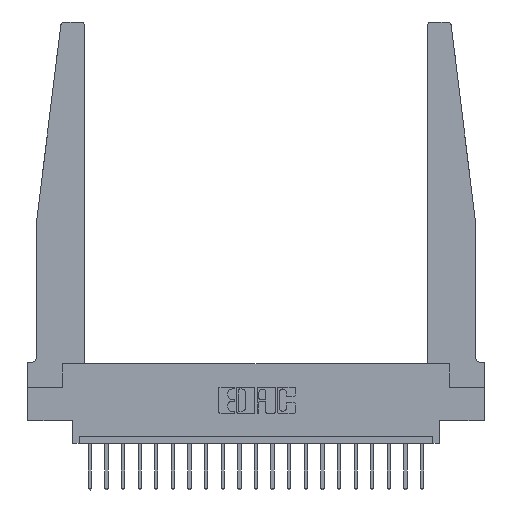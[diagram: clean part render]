
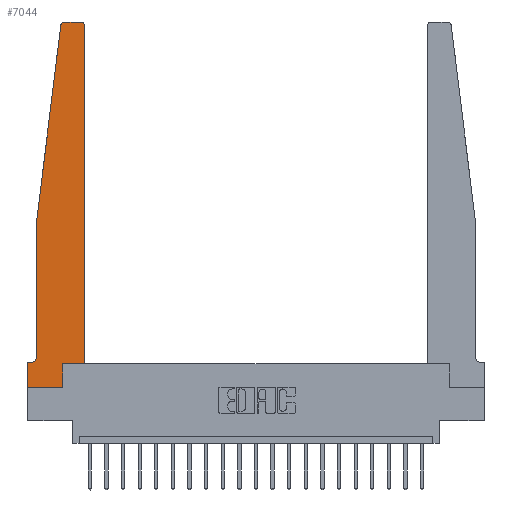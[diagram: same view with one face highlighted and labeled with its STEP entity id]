
A CAD part, top view. The second image highlights one B-rep face of the part: STEP entity #7044.
In plain terms, the highlighted planar face has unit normal (0, 0, 1).
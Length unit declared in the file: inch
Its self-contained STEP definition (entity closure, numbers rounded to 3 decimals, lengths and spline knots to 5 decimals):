
#80 = DIRECTION ( 'NONE',  ( 1., 0., 0. ) ) ;
#174 = VECTOR ( 'NONE', #80, 39.37008 ) ;
#444 = EDGE_CURVE ( 'NONE', #9945, #9003, #4752, .T. ) ;
#501 = CARTESIAN_POINT ( 'NONE',  ( 0.425, 0.18, 0.37 ) ) ;
#555 = EDGE_CURVE ( 'NONE', #20410, #11046, #13767, .T. ) ;
#638 = ORIENTED_EDGE ( 'NONE', *, *, #2911, .T. ) ;
#1196 = DIRECTION ( 'NONE',  ( -1., 0., 0. ) ) ;
#1366 = CIRCLE ( 'NONE', #17607, 0.05 ) ;
#1456 = EDGE_CURVE ( 'NONE', #18994, #9248, #15527, .T. ) ;
#1586 = CARTESIAN_POINT ( 'NONE',  ( 0.015, 0.2375, 0.37 ) ) ;
#1718 = CARTESIAN_POINT ( 'NONE',  ( 0.2605, 0.18, 0.37 ) ) ;
#1990 = DIRECTION ( 'NONE',  ( 0., 0., 1. ) ) ;
#2116 = CARTESIAN_POINT ( 'NONE',  ( 0.065, 1.25, 0.37 ) ) ;
#2393 = LINE ( 'NONE', #12833, #174 ) ;
#2533 = EDGE_CURVE ( 'NONE', #6152, #16121, #2393, .T. ) ;
#2654 = CARTESIAN_POINT ( 'NONE',  ( 0.065, 0.2375, 0.37 ) ) ;
#2911 = EDGE_CURVE ( 'NONE', #16121, #20410, #12170, .T. ) ;
#3123 = DIRECTION ( 'NONE',  ( 0., 1., 0. ) ) ;
#3653 = CARTESIAN_POINT ( 'NONE',  ( 0.27653, 2.75, 0.37 ) ) ;
#4522 = EDGE_CURVE ( 'NONE', #17151, #15893, #19498, .T. ) ;
#4752 = LINE ( 'NONE', #17901, #18113 ) ;
#4829 = ORIENTED_EDGE ( 'NONE', *, *, #555, .T. ) ;
#5162 = CARTESIAN_POINT ( 'NONE',  ( 0.2605, 0.18, 0.37 ) ) ;
#5290 = ORIENTED_EDGE ( 'NONE', *, *, #2533, .T. ) ;
#6021 = ORIENTED_EDGE ( 'NONE', *, *, #19096, .T. ) ;
#6152 = VERTEX_POINT ( 'NONE', #19234 ) ;
#6263 = CARTESIAN_POINT ( 'NONE',  ( 0.425, 0.18, 0.37 ) ) ;
#6831 = DIRECTION ( 'NONE',  ( 0., 0., 1. ) ) ;
#7044 = ADVANCED_FACE ( 'NONE', ( #10364 ), #8907, .T. ) ;
#7380 = CARTESIAN_POINT ( 'NONE',  ( 0.27653, 2.72, 0.37 ) ) ;
#7527 = LINE ( 'NONE', #7545, #18342 ) ;
#7545 = CARTESIAN_POINT ( 'NONE',  ( 0.065, 0.1875, 0.37 ) ) ;
#7859 = ORIENTED_EDGE ( 'NONE', *, *, #19901, .T. ) ;
#7896 = VECTOR ( 'NONE', #3123, 39.37008 ) ;
#8209 = CARTESIAN_POINT ( 'NONE',  ( 0.425, 2.72, 0.37 ) ) ;
#8260 = VERTEX_POINT ( 'NONE', #8263 ) ;
#8263 = CARTESIAN_POINT ( 'NONE',  ( 0.015, 0.1875, 0.37 ) ) ;
#8597 = EDGE_CURVE ( 'NONE', #8260, #12602, #7527, .T. ) ;
#8748 = CARTESIAN_POINT ( 'NONE',  ( 0., 0., 0.37 ) ) ;
#8907 = PLANE ( 'NONE',  #12586 ) ;
#8940 = DIRECTION ( 'NONE',  ( 0., 0., 1. ) ) ;
#9003 = VERTEX_POINT ( 'NONE', #2654 ) ;
#9209 = CARTESIAN_POINT ( 'NONE',  ( 0.25, 2.75, 0.37 ) ) ;
#9248 = VERTEX_POINT ( 'NONE', #9755 ) ;
#9514 = EDGE_CURVE ( 'NONE', #12602, #6152, #20285, .T. ) ;
#9755 = CARTESIAN_POINT ( 'NONE',  ( 0.24675, 2.72367, 0.37 ) ) ;
#9798 = DIRECTION ( 'NONE',  ( 0., -1., 0. ) ) ;
#9866 = DIRECTION ( 'NONE',  ( 1., 0., 0. ) ) ;
#9945 = VERTEX_POINT ( 'NONE', #17171 ) ;
#9972 = DIRECTION ( 'NONE',  ( 0., 1., 0. ) ) ;
#10186 = EDGE_LOOP ( 'NONE', ( #12914, #20070, #19013, #15661, #7859, #15151, #16460, #5290, #638, #4829, #6021, #18436 ) ) ;
#10364 = FACE_OUTER_BOUND ( 'NONE', #10186, .T. ) ;
#10478 = DIRECTION ( 'NONE',  ( 1., 0., 0. ) ) ;
#10799 = LINE ( 'NONE', #9209, #13544 ) ;
#11043 = DIRECTION ( 'NONE',  ( -1., 0., 0. ) ) ;
#11046 = VERTEX_POINT ( 'NONE', #6263 ) ;
#11756 = VECTOR ( 'NONE', #20038, 39.37008 ) ;
#11877 = DIRECTION ( 'NONE',  ( -0.122, -0.992, 0. ) ) ;
#12170 = LINE ( 'NONE', #5162, #7896 ) ;
#12271 = CARTESIAN_POINT ( 'NONE',  ( 0., 0.1875, 0.37 ) ) ;
#12455 = LINE ( 'NONE', #501, #16519 ) ;
#12586 = AXIS2_PLACEMENT_3D ( 'NONE', #12271, #6831, #13400 ) ;
#12602 = VERTEX_POINT ( 'NONE', #15111 ) ;
#12833 = CARTESIAN_POINT ( 'NONE',  ( 0., 0., 0.37 ) ) ;
#12914 = ORIENTED_EDGE ( 'NONE', *, *, #16598, .T. ) ;
#13043 = DIRECTION ( 'NONE',  ( 0., 0., -1. ) ) ;
#13400 = DIRECTION ( 'NONE',  ( 1., 0., 0. ) ) ;
#13544 = VECTOR ( 'NONE', #1196, 39.37008 ) ;
#13767 = LINE ( 'NONE', #14600, #18095 ) ;
#13992 = CARTESIAN_POINT ( 'NONE',  ( 0.395, 2.75, 0.37 ) ) ;
#14600 = CARTESIAN_POINT ( 'NONE',  ( 0.425, 0.18, 0.37 ) ) ;
#15084 = AXIS2_PLACEMENT_3D ( 'NONE', #7380, #8940, #10478 ) ;
#15111 = CARTESIAN_POINT ( 'NONE',  ( 0., 0.1875, 0.37 ) ) ;
#15151 = ORIENTED_EDGE ( 'NONE', *, *, #8597, .T. ) ;
#15527 = CIRCLE ( 'NONE', #15084, 0.03 ) ;
#15661 = ORIENTED_EDGE ( 'NONE', *, *, #444, .T. ) ;
#15893 = VERTEX_POINT ( 'NONE', #13992 ) ;
#16121 = VERTEX_POINT ( 'NONE', #20650 ) ;
#16460 = ORIENTED_EDGE ( 'NONE', *, *, #9514, .T. ) ;
#16519 = VECTOR ( 'NONE', #9972, 39.37008 ) ;
#16598 = EDGE_CURVE ( 'NONE', #15893, #18994, #10799, .T. ) ;
#17151 = VERTEX_POINT ( 'NONE', #8209 ) ;
#17171 = CARTESIAN_POINT ( 'NONE',  ( 0.065, 1.25, 0.37 ) ) ;
#17607 = AXIS2_PLACEMENT_3D ( 'NONE', #1586, #13043, #19210 ) ;
#17881 = DIRECTION ( 'NONE',  ( 1., 0., 0. ) ) ;
#17901 = CARTESIAN_POINT ( 'NONE',  ( 0.065, 1.25, 0.37 ) ) ;
#18095 = VECTOR ( 'NONE', #17881, 39.37008 ) ;
#18113 = VECTOR ( 'NONE', #9798, 39.37008 ) ;
#18342 = VECTOR ( 'NONE', #11043, 39.37008 ) ;
#18436 = ORIENTED_EDGE ( 'NONE', *, *, #4522, .T. ) ;
#18571 = EDGE_CURVE ( 'NONE', #9248, #9945, #20263, .T. ) ;
#18994 = VERTEX_POINT ( 'NONE', #3653 ) ;
#19013 = ORIENTED_EDGE ( 'NONE', *, *, #18571, .T. ) ;
#19096 = EDGE_CURVE ( 'NONE', #11046, #17151, #12455, .T. ) ;
#19210 = DIRECTION ( 'NONE',  ( -1., 0., 0. ) ) ;
#19234 = CARTESIAN_POINT ( 'NONE',  ( 0., 0., 0.37 ) ) ;
#19466 = CARTESIAN_POINT ( 'NONE',  ( 0.395, 2.72, 0.37 ) ) ;
#19498 = CIRCLE ( 'NONE', #20360, 0.03 ) ;
#19901 = EDGE_CURVE ( 'NONE', #9003, #8260, #1366, .T. ) ;
#20038 = DIRECTION ( 'NONE',  ( 0., -1., 0. ) ) ;
#20070 = ORIENTED_EDGE ( 'NONE', *, *, #1456, .T. ) ;
#20263 = LINE ( 'NONE', #2116, #20520 ) ;
#20285 = LINE ( 'NONE', #8748, #11756 ) ;
#20360 = AXIS2_PLACEMENT_3D ( 'NONE', #19466, #1990, #9866 ) ;
#20410 = VERTEX_POINT ( 'NONE', #1718 ) ;
#20520 = VECTOR ( 'NONE', #11877, 39.37008 ) ;
#20650 = CARTESIAN_POINT ( 'NONE',  ( 0.2605, 0., 0.37 ) ) ;
